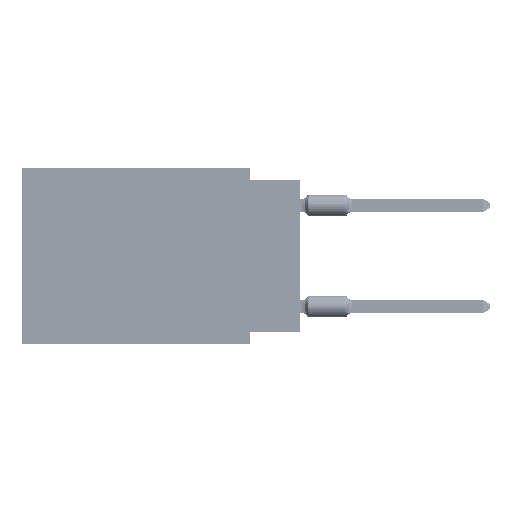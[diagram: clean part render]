
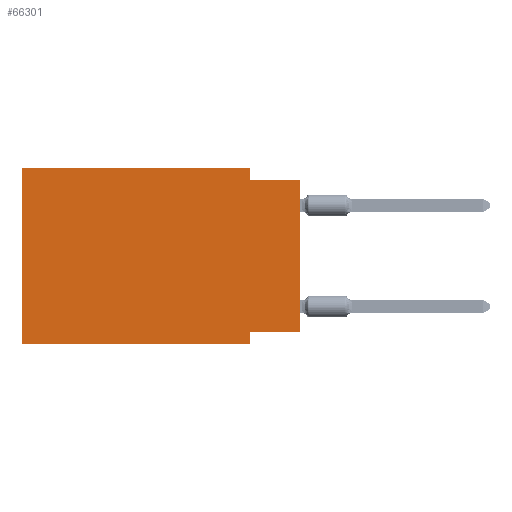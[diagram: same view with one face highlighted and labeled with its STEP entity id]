
A CAD part, left-side view. The second image highlights one B-rep face of the part: STEP entity #66301.
In plain terms, the highlighted planar face has unit normal (-1, 0, 0).
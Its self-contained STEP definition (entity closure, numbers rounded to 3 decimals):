
#562 = ORIENTED_EDGE ( 'NONE', *, *, #93046, .F. ) ;
#4117 = DIRECTION ( 'NONE',  ( 0., -1., 0. ) ) ;
#6305 = LINE ( 'NONE', #93202, #58378 ) ;
#7492 = DIRECTION ( 'NONE',  ( 0., 0., -1. ) ) ;
#7991 = VECTOR ( 'NONE', #32569, 1000. ) ;
#8694 = AXIS2_PLACEMENT_3D ( 'NONE', #15065, #35536, #7492 ) ;
#9128 = CARTESIAN_POINT ( 'NONE',  ( 0., 13.97, -8.89 ) ) ;
#9567 = VERTEX_POINT ( 'NONE', #90034 ) ;
#9853 = ORIENTED_EDGE ( 'NONE', *, *, #61364, .T. ) ;
#10982 = CARTESIAN_POINT ( 'NONE',  ( 0., 2.54, -8.255 ) ) ;
#11745 = VERTEX_POINT ( 'NONE', #10982 ) ;
#15065 = CARTESIAN_POINT ( 'NONE',  ( 0., 13.97, 0. ) ) ;
#17160 = DIRECTION ( 'NONE',  ( 0., 0., -1. ) ) ;
#17539 = CARTESIAN_POINT ( 'NONE',  ( 0., 0., 0. ) ) ;
#18559 = CARTESIAN_POINT ( 'NONE',  ( 0., 0., -0.635 ) ) ;
#18643 = DIRECTION ( 'NONE',  ( 0., 1., 0. ) ) ;
#19046 = LINE ( 'NONE', #18559, #40441 ) ;
#19187 = VERTEX_POINT ( 'NONE', #55361 ) ;
#20342 = PLANE ( 'NONE',  #8694 ) ;
#21949 = EDGE_CURVE ( 'NONE', #54983, #77794, #6305, .T. ) ;
#23100 = LINE ( 'NONE', #39248, #7991 ) ;
#24792 = CARTESIAN_POINT ( 'NONE',  ( 0., 2.54, -0.635 ) ) ;
#26081 = ORIENTED_EDGE ( 'NONE', *, *, #69205, .T. ) ;
#31645 = EDGE_CURVE ( 'NONE', #57265, #19187, #23100, .T. ) ;
#32569 = DIRECTION ( 'NONE',  ( 0., 0., 1. ) ) ;
#32627 = LINE ( 'NONE', #46892, #51841 ) ;
#32936 = LINE ( 'NONE', #83683, #36682 ) ;
#34265 = CARTESIAN_POINT ( 'NONE',  ( 0., 2.54, -8.89 ) ) ;
#35536 = DIRECTION ( 'NONE',  ( 1., 0., 0. ) ) ;
#36682 = VECTOR ( 'NONE', #18643, 1000. ) ;
#37478 = ORIENTED_EDGE ( 'NONE', *, *, #65672, .F. ) ;
#39248 = CARTESIAN_POINT ( 'NONE',  ( 0., 13.97, 0. ) ) ;
#40441 = VECTOR ( 'NONE', #70311, 1000. ) ;
#40733 = VECTOR ( 'NONE', #58447, 1000. ) ;
#42809 = LINE ( 'NONE', #86470, #40733 ) ;
#46892 = CARTESIAN_POINT ( 'NONE',  ( 0., 13.97, 0. ) ) ;
#47668 = EDGE_CURVE ( 'NONE', #92698, #11745, #32936, .T. ) ;
#47921 = LINE ( 'NONE', #17539, #70394 ) ;
#49700 = ORIENTED_EDGE ( 'NONE', *, *, #47668, .F. ) ;
#49948 = EDGE_CURVE ( 'NONE', #19187, #54983, #32627, .T. ) ;
#51841 = VECTOR ( 'NONE', #4117, 1000. ) ;
#54983 = VERTEX_POINT ( 'NONE', #63356 ) ;
#55361 = CARTESIAN_POINT ( 'NONE',  ( 0., 13.97, 0. ) ) ;
#57265 = VERTEX_POINT ( 'NONE', #9128 ) ;
#57460 = VERTEX_POINT ( 'NONE', #34265 ) ;
#58378 = VECTOR ( 'NONE', #17160, 1000. ) ;
#58447 = DIRECTION ( 'NONE',  ( 0., 0., -1. ) ) ;
#59439 = CARTESIAN_POINT ( 'NONE',  ( 0., 13.97, -8.89 ) ) ;
#60398 = LINE ( 'NONE', #59439, #78883 ) ;
#61364 = EDGE_CURVE ( 'NONE', #92698, #9567, #47921, .T. ) ;
#63356 = CARTESIAN_POINT ( 'NONE',  ( 0., 2.54, 0. ) ) ;
#65644 = DIRECTION ( 'NONE',  ( 0., -1., 0. ) ) ;
#65672 = EDGE_CURVE ( 'NONE', #77794, #9567, #19046, .T. ) ;
#66301 = ADVANCED_FACE ( 'NONE', ( #85362 ), #20342, .F. ) ;
#69205 = EDGE_CURVE ( 'NONE', #57265, #57460, #60398, .T. ) ;
#70311 = DIRECTION ( 'NONE',  ( 0., -1., 0. ) ) ;
#70394 = VECTOR ( 'NONE', #82119, 1000. ) ;
#76117 = ORIENTED_EDGE ( 'NONE', *, *, #21949, .F. ) ;
#77794 = VERTEX_POINT ( 'NONE', #24792 ) ;
#78883 = VECTOR ( 'NONE', #65644, 1000. ) ;
#79385 = ORIENTED_EDGE ( 'NONE', *, *, #49948, .F. ) ;
#82119 = DIRECTION ( 'NONE',  ( 0., 0., 1. ) ) ;
#83683 = CARTESIAN_POINT ( 'NONE',  ( 0., 0., -8.255 ) ) ;
#84038 = ORIENTED_EDGE ( 'NONE', *, *, #31645, .F. ) ;
#85362 = FACE_OUTER_BOUND ( 'NONE', #92890, .T. ) ;
#86470 = CARTESIAN_POINT ( 'NONE',  ( 0., 2.54, -8.89 ) ) ;
#90034 = CARTESIAN_POINT ( 'NONE',  ( 0., 0., -0.635 ) ) ;
#90321 = CARTESIAN_POINT ( 'NONE',  ( 0., 0., -8.255 ) ) ;
#92698 = VERTEX_POINT ( 'NONE', #90321 ) ;
#92890 = EDGE_LOOP ( 'NONE', ( #9853, #37478, #76117, #79385, #84038, #26081, #562, #49700 ) ) ;
#93046 = EDGE_CURVE ( 'NONE', #11745, #57460, #42809, .T. ) ;
#93202 = CARTESIAN_POINT ( 'NONE',  ( 0., 2.54, 0. ) ) ;
